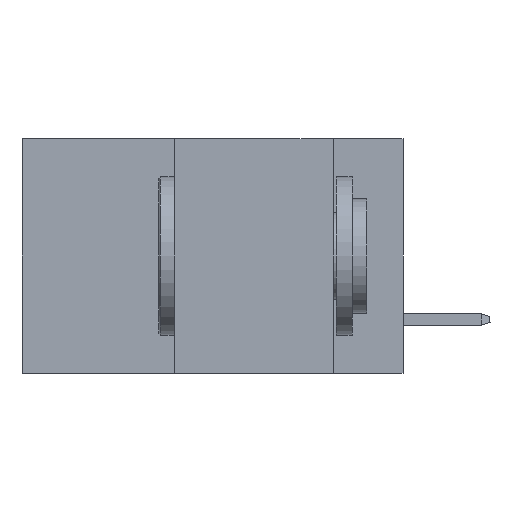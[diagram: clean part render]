
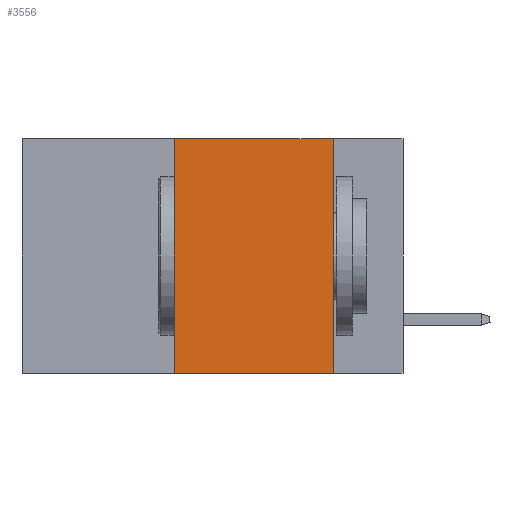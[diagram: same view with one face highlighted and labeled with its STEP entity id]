
A CAD part, left-side view. The second image highlights one B-rep face of the part: STEP entity #3556.
In plain terms, the highlighted planar face has unit normal (-1, 0, 0).
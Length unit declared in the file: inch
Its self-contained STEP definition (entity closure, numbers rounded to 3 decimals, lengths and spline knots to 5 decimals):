
#356 = DIRECTION ( 'NONE',  ( 0., 0., -1. ) ) ;
#1638 = DIRECTION ( 'NONE',  ( 0., -1., 0. ) ) ;
#1842 = EDGE_CURVE ( 'NONE', #20301, #11999, #9400, .T. ) ;
#1982 = CARTESIAN_POINT ( 'NONE',  ( 0., 0.6, 0. ) ) ;
#2851 = CARTESIAN_POINT ( 'NONE',  ( 0., 0.11, 0. ) ) ;
#3556 = ADVANCED_FACE ( 'NONE', ( #13465 ), #20875, .F. ) ;
#4628 = EDGE_CURVE ( 'NONE', #22965, #20301, #6346, .T. ) ;
#6057 = CARTESIAN_POINT ( 'NONE',  ( 0., 0.36, -0.37 ) ) ;
#6346 = LINE ( 'NONE', #21181, #9848 ) ;
#6583 = VECTOR ( 'NONE', #22992, 39.37008 ) ;
#7918 = EDGE_LOOP ( 'NONE', ( #17168, #23096, #20966, #7975 ) ) ;
#7975 = ORIENTED_EDGE ( 'NONE', *, *, #12524, .T. ) ;
#8176 = DIRECTION ( 'NONE',  ( 0., 0., -1. ) ) ;
#9400 = LINE ( 'NONE', #1982, #6583 ) ;
#9848 = VECTOR ( 'NONE', #15646, 39.37008 ) ;
#10130 = AXIS2_PLACEMENT_3D ( 'NONE', #16940, #20999, #356 ) ;
#10319 = CARTESIAN_POINT ( 'NONE',  ( 0., 0.36, 0. ) ) ;
#10771 = CARTESIAN_POINT ( 'NONE',  ( 0., 0.6, -0.37 ) ) ;
#10875 = VERTEX_POINT ( 'NONE', #19694 ) ;
#11117 = VECTOR ( 'NONE', #8176, 39.37008 ) ;
#11999 = VERTEX_POINT ( 'NONE', #18996 ) ;
#12524 = EDGE_CURVE ( 'NONE', #22965, #10875, #18233, .T. ) ;
#12867 = EDGE_CURVE ( 'NONE', #11999, #10875, #14133, .T. ) ;
#13465 = FACE_OUTER_BOUND ( 'NONE', #7918, .T. ) ;
#14133 = LINE ( 'NONE', #2851, #11117 ) ;
#14686 = VECTOR ( 'NONE', #1638, 39.37008 ) ;
#15646 = DIRECTION ( 'NONE',  ( 0., 0., 1. ) ) ;
#16940 = CARTESIAN_POINT ( 'NONE',  ( 0., 0.6, 0. ) ) ;
#17168 = ORIENTED_EDGE ( 'NONE', *, *, #12867, .F. ) ;
#18233 = LINE ( 'NONE', #10771, #14686 ) ;
#18996 = CARTESIAN_POINT ( 'NONE',  ( 0., 0.11, 0. ) ) ;
#19694 = CARTESIAN_POINT ( 'NONE',  ( 0., 0.11, -0.37 ) ) ;
#20301 = VERTEX_POINT ( 'NONE', #10319 ) ;
#20875 = PLANE ( 'NONE',  #10130 ) ;
#20966 = ORIENTED_EDGE ( 'NONE', *, *, #4628, .F. ) ;
#20999 = DIRECTION ( 'NONE',  ( 1., 0., 0. ) ) ;
#21181 = CARTESIAN_POINT ( 'NONE',  ( 0., 0.36, 0. ) ) ;
#22965 = VERTEX_POINT ( 'NONE', #6057 ) ;
#22992 = DIRECTION ( 'NONE',  ( 0., -1., 0. ) ) ;
#23096 = ORIENTED_EDGE ( 'NONE', *, *, #1842, .F. ) ;
